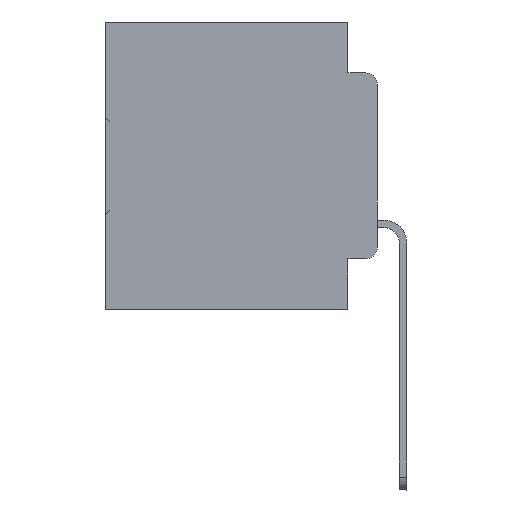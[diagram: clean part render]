
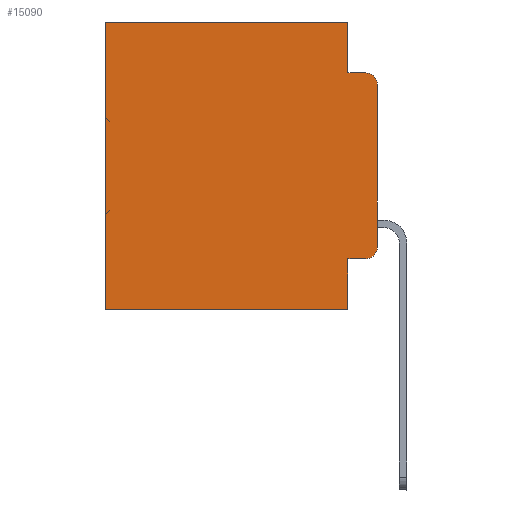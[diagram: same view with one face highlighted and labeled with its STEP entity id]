
A CAD part, left-side view. The second image highlights one B-rep face of the part: STEP entity #15090.
In plain terms, the highlighted planar face has unit normal (-1, 0, 0).
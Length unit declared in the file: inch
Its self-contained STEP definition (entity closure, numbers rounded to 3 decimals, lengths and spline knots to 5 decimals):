
#209 = DIRECTION ( 'NONE',  ( 0., -1., 0. ) ) ;
#471 = LINE ( 'NONE', #16514, #17657 ) ;
#505 = AXIS2_PLACEMENT_3D ( 'NONE', #2750, #19262, #36412 ) ;
#943 = DIRECTION ( 'NONE',  ( 0., 0., -1. ) ) ;
#1001 = CARTESIAN_POINT ( 'NONE',  ( 0.298, 0., -0.1085 ) ) ;
#1766 = VECTOR ( 'NONE', #5141, 39.37008 ) ;
#1795 = VERTEX_POINT ( 'NONE', #1001 ) ;
#2750 = CARTESIAN_POINT ( 'NONE',  ( 0.298, 0., 0. ) ) ;
#2866 = LINE ( 'NONE', #23183, #4651 ) ;
#2981 = CARTESIAN_POINT ( 'NONE',  ( 0.298, 0.473, 0. ) ) ;
#3001 = ORIENTED_EDGE ( 'NONE', *, *, #30671, .F. ) ;
#3123 = VECTOR ( 'NONE', #943, 39.37008 ) ;
#3480 = ORIENTED_EDGE ( 'NONE', *, *, #8944, .T. ) ;
#3724 = VECTOR ( 'NONE', #28371, 39.37008 ) ;
#4651 = VECTOR ( 'NONE', #6311, 39.37008 ) ;
#5141 = DIRECTION ( 'NONE',  ( 0., 0., -1. ) ) ;
#5479 = ORIENTED_EDGE ( 'NONE', *, *, #21123, .T. ) ;
#5512 = VERTEX_POINT ( 'NONE', #19254 ) ;
#6280 = CARTESIAN_POINT ( 'NONE',  ( 0.298, 0.051, -0.5 ) ) ;
#6311 = DIRECTION ( 'NONE',  ( 0., 1., 0. ) ) ;
#6580 = EDGE_CURVE ( 'NONE', #1795, #11812, #33131, .T. ) ;
#6921 = VERTEX_POINT ( 'NONE', #26175 ) ;
#7115 = EDGE_CURVE ( 'NONE', #33721, #6921, #20291, .T. ) ;
#8297 = PLANE ( 'NONE',  #505 ) ;
#8475 = LINE ( 'NONE', #15107, #3123 ) ;
#8496 = CARTESIAN_POINT ( 'NONE',  ( 0.298, 0.051, -0.0885 ) ) ;
#8861 = FACE_OUTER_BOUND ( 'NONE', #10234, .T. ) ;
#8944 = EDGE_CURVE ( 'NONE', #5512, #33721, #471, .T. ) ;
#9135 = VERTEX_POINT ( 'NONE', #22665 ) ;
#9239 = EDGE_CURVE ( 'NONE', #5512, #30064, #8475, .T. ) ;
#9253 = ORIENTED_EDGE ( 'NONE', *, *, #24115, .F. ) ;
#9880 = LINE ( 'NONE', #11481, #3724 ) ;
#10085 = EDGE_CURVE ( 'NONE', #1795, #6921, #31310, .T. ) ;
#10097 = CARTESIAN_POINT ( 'NONE',  ( 0.298, 0.473, 0. ) ) ;
#10234 = EDGE_LOOP ( 'NONE', ( #18093, #10556, #9253, #3001, #27863, #5479, #19878, #10440, #3480, #20779 ) ) ;
#10440 = ORIENTED_EDGE ( 'NONE', *, *, #9239, .F. ) ;
#10556 = ORIENTED_EDGE ( 'NONE', *, *, #6580, .T. ) ;
#11481 = CARTESIAN_POINT ( 'NONE',  ( 0.298, 0., 0. ) ) ;
#11812 = VERTEX_POINT ( 'NONE', #33818 ) ;
#12146 = CARTESIAN_POINT ( 'NONE',  ( 0.298, 0.051, 0. ) ) ;
#13347 = EDGE_CURVE ( 'NONE', #29015, #15250, #9880, .T. ) ;
#13919 = DIRECTION ( 'NONE',  ( 0., -1., 0. ) ) ;
#14956 = DIRECTION ( 'NONE',  ( 0., 0., -1. ) ) ;
#15090 = ADVANCED_FACE ( 'NONE', ( #8861 ), #8297, .F. ) ;
#15107 = CARTESIAN_POINT ( 'NONE',  ( 0.298, 0.051, 0. ) ) ;
#15187 = CARTESIAN_POINT ( 'NONE',  ( 0.298, 0.02, -0.3915 ) ) ;
#15213 = CARTESIAN_POINT ( 'NONE',  ( 0.298, 0.473, -0.5 ) ) ;
#15250 = VERTEX_POINT ( 'NONE', #2981 ) ;
#15898 = AXIS2_PLACEMENT_3D ( 'NONE', #35481, #18804, #21266 ) ;
#16406 = VECTOR ( 'NONE', #29558, 39.37008 ) ;
#16514 = CARTESIAN_POINT ( 'NONE',  ( 0.298, 0.051, -0.4115 ) ) ;
#17281 = AXIS2_PLACEMENT_3D ( 'NONE', #15187, #24076, #18275 ) ;
#17657 = VECTOR ( 'NONE', #13919, 39.37008 ) ;
#18093 = ORIENTED_EDGE ( 'NONE', *, *, #10085, .F. ) ;
#18275 = DIRECTION ( 'NONE',  ( 0., 0., -1. ) ) ;
#18804 = DIRECTION ( 'NONE',  ( -1., 0., 0. ) ) ;
#18977 = EDGE_CURVE ( 'NONE', #30064, #32344, #2866, .T. ) ;
#19254 = CARTESIAN_POINT ( 'NONE',  ( 0.298, 0.051, -0.4115 ) ) ;
#19262 = DIRECTION ( 'NONE',  ( 1., 0., 0. ) ) ;
#19878 = ORIENTED_EDGE ( 'NONE', *, *, #18977, .F. ) ;
#20291 = CIRCLE ( 'NONE', #17281, 0.02 ) ;
#20779 = ORIENTED_EDGE ( 'NONE', *, *, #7115, .T. ) ;
#21123 = EDGE_CURVE ( 'NONE', #15250, #32344, #33187, .T. ) ;
#21266 = DIRECTION ( 'NONE',  ( 0., 0., -1. ) ) ;
#21995 = CARTESIAN_POINT ( 'NONE',  ( 0.298, 0., 0. ) ) ;
#22665 = CARTESIAN_POINT ( 'NONE',  ( 0.298, 0.051, -0.0885 ) ) ;
#23183 = CARTESIAN_POINT ( 'NONE',  ( 0.298, 0., -0.5 ) ) ;
#24076 = DIRECTION ( 'NONE',  ( -1., 0., 0. ) ) ;
#24115 = EDGE_CURVE ( 'NONE', #9135, #11812, #33764, .T. ) ;
#26175 = CARTESIAN_POINT ( 'NONE',  ( 0.298, 0., -0.3915 ) ) ;
#26302 = LINE ( 'NONE', #12146, #29364 ) ;
#27863 = ORIENTED_EDGE ( 'NONE', *, *, #13347, .T. ) ;
#28371 = DIRECTION ( 'NONE',  ( 0., 1., 0. ) ) ;
#29015 = VERTEX_POINT ( 'NONE', #33848 ) ;
#29364 = VECTOR ( 'NONE', #14956, 39.37008 ) ;
#29558 = DIRECTION ( 'NONE',  ( 0., 0., -1. ) ) ;
#30064 = VERTEX_POINT ( 'NONE', #6280 ) ;
#30671 = EDGE_CURVE ( 'NONE', #29015, #9135, #26302, .T. ) ;
#31100 = VECTOR ( 'NONE', #209, 39.37008 ) ;
#31310 = LINE ( 'NONE', #21995, #1766 ) ;
#32344 = VERTEX_POINT ( 'NONE', #15213 ) ;
#33131 = CIRCLE ( 'NONE', #15898, 0.02 ) ;
#33187 = LINE ( 'NONE', #10097, #16406 ) ;
#33721 = VERTEX_POINT ( 'NONE', #35601 ) ;
#33764 = LINE ( 'NONE', #8496, #31100 ) ;
#33818 = CARTESIAN_POINT ( 'NONE',  ( 0.298, 0.02, -0.0885 ) ) ;
#33848 = CARTESIAN_POINT ( 'NONE',  ( 0.298, 0.051, 0. ) ) ;
#35481 = CARTESIAN_POINT ( 'NONE',  ( 0.298, 0.02, -0.1085 ) ) ;
#35601 = CARTESIAN_POINT ( 'NONE',  ( 0.298, 0.02, -0.4115 ) ) ;
#36412 = DIRECTION ( 'NONE',  ( 0., 0., -1. ) ) ;
